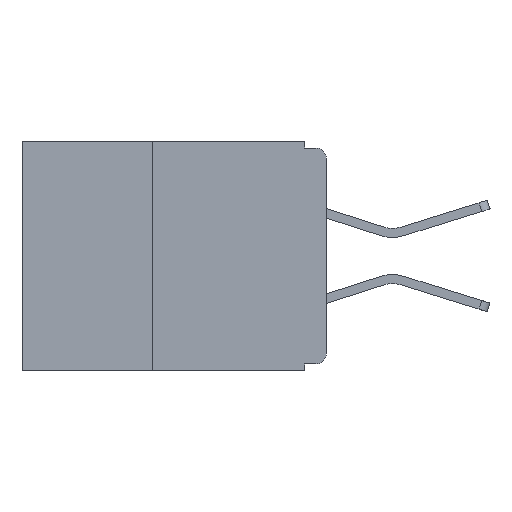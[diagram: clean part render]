
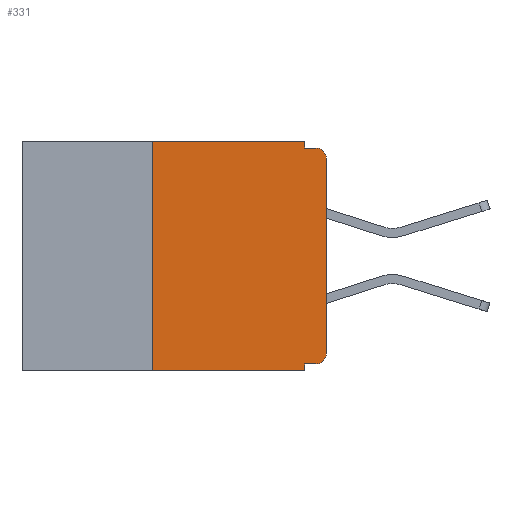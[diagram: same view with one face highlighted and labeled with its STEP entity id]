
A CAD part, left-side view. The second image highlights one B-rep face of the part: STEP entity #331.
In plain terms, the highlighted planar face has unit normal (-1, 0, 0).
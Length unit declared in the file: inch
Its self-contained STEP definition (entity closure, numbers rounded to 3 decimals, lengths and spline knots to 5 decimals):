
#97 = ORIENTED_EDGE ( 'NONE', *, *, #522, .F. ) ;
#331 = ADVANCED_FACE ( 'NONE', ( #19796 ), #12678, .F. ) ;
#342 = ORIENTED_EDGE ( 'NONE', *, *, #9798, .T. ) ;
#350 = VECTOR ( 'NONE', #2283, 39.37008 ) ;
#358 = EDGE_LOOP ( 'NONE', ( #603, #11187, #97, #20735, #12195, #6514, #342, #10022, #10660, #18268 ) ) ;
#522 = EDGE_CURVE ( 'NONE', #19656, #4964, #21245, .T. ) ;
#603 = ORIENTED_EDGE ( 'NONE', *, *, #3829, .T. ) ;
#1118 = CARTESIAN_POINT ( 'NONE',  ( 0., 0., -0.32 ) ) ;
#2044 = VECTOR ( 'NONE', #4149, 39.37008 ) ;
#2244 = CARTESIAN_POINT ( 'NONE',  ( 0., 0.25, -0.33 ) ) ;
#2283 = DIRECTION ( 'NONE',  ( 0., 0., -1. ) ) ;
#2284 = VERTEX_POINT ( 'NONE', #16833 ) ;
#2367 = VECTOR ( 'NONE', #20820, 39.37008 ) ;
#2995 = DIRECTION ( 'NONE',  ( 0., 1., 0. ) ) ;
#3829 = EDGE_CURVE ( 'NONE', #8977, #16353, #7368, .T. ) ;
#3917 = CARTESIAN_POINT ( 'NONE',  ( 0., 0.015, -0.305 ) ) ;
#4149 = DIRECTION ( 'NONE',  ( 0., 0., 1. ) ) ;
#4964 = VERTEX_POINT ( 'NONE', #22934 ) ;
#5152 = VECTOR ( 'NONE', #16269, 39.37008 ) ;
#5301 = VERTEX_POINT ( 'NONE', #5804 ) ;
#5392 = CARTESIAN_POINT ( 'NONE',  ( 0., 0.031, 0. ) ) ;
#5720 = LINE ( 'NONE', #10609, #20074 ) ;
#5778 = DIRECTION ( 'NONE',  ( 0., 0., -1. ) ) ;
#5804 = CARTESIAN_POINT ( 'NONE',  ( 0., 0.031, -0.33 ) ) ;
#5842 = CARTESIAN_POINT ( 'NONE',  ( 0., 0., -0.025 ) ) ;
#6514 = ORIENTED_EDGE ( 'NONE', *, *, #10430, .F. ) ;
#6812 = EDGE_CURVE ( 'NONE', #2284, #11528, #15078, .T. ) ;
#7368 = LINE ( 'NONE', #10387, #16692 ) ;
#7522 = VERTEX_POINT ( 'NONE', #18755 ) ;
#7772 = CARTESIAN_POINT ( 'NONE',  ( 0., 0.437, -0.33 ) ) ;
#8536 = CARTESIAN_POINT ( 'NONE',  ( 0., 0.015, -0.025 ) ) ;
#8763 = DIRECTION ( 'NONE',  ( 0., 0., -1. ) ) ;
#8977 = VERTEX_POINT ( 'NONE', #22898 ) ;
#9481 = EDGE_CURVE ( 'NONE', #16353, #4964, #14965, .T. ) ;
#9701 = VERTEX_POINT ( 'NONE', #12780 ) ;
#9798 = EDGE_CURVE ( 'NONE', #17469, #5301, #12342, .T. ) ;
#9914 = DIRECTION ( 'NONE',  ( 0., 0., -1. ) ) ;
#9920 = DIRECTION ( 'NONE',  ( 1., 0., 0. ) ) ;
#10022 = ORIENTED_EDGE ( 'NONE', *, *, #15241, .F. ) ;
#10387 = CARTESIAN_POINT ( 'NONE',  ( 0., 0., 0. ) ) ;
#10406 = DIRECTION ( 'NONE',  ( 0., 0., -1. ) ) ;
#10430 = EDGE_CURVE ( 'NONE', #17469, #2284, #16940, .T. ) ;
#10609 = CARTESIAN_POINT ( 'NONE',  ( 0., 0.031, 0. ) ) ;
#10660 = ORIENTED_EDGE ( 'NONE', *, *, #12763, .F. ) ;
#11187 = ORIENTED_EDGE ( 'NONE', *, *, #9481, .T. ) ;
#11346 = VECTOR ( 'NONE', #18023, 39.37008 ) ;
#11528 = VERTEX_POINT ( 'NONE', #5392 ) ;
#12195 = ORIENTED_EDGE ( 'NONE', *, *, #6812, .F. ) ;
#12342 = LINE ( 'NONE', #7772, #2367 ) ;
#12678 = PLANE ( 'NONE',  #18622 ) ;
#12763 = EDGE_CURVE ( 'NONE', #7522, #9701, #21228, .T. ) ;
#12780 = CARTESIAN_POINT ( 'NONE',  ( 0., 0.031, -0.32 ) ) ;
#12805 = EDGE_CURVE ( 'NONE', #11528, #19656, #5720, .T. ) ;
#14474 = CARTESIAN_POINT ( 'NONE',  ( 0., 0.437, 0. ) ) ;
#14965 = CIRCLE ( 'NONE', #21642, 0.015 ) ;
#15078 = LINE ( 'NONE', #14474, #5152 ) ;
#15241 = EDGE_CURVE ( 'NONE', #9701, #5301, #20256, .T. ) ;
#16269 = DIRECTION ( 'NONE',  ( 0., -1., 0. ) ) ;
#16331 = CARTESIAN_POINT ( 'NONE',  ( 0., 0.437, 0. ) ) ;
#16353 = VERTEX_POINT ( 'NONE', #5842 ) ;
#16692 = VECTOR ( 'NONE', #21546, 39.37008 ) ;
#16795 = CIRCLE ( 'NONE', #17364, 0.015 ) ;
#16833 = CARTESIAN_POINT ( 'NONE',  ( 0., 0.25, 0. ) ) ;
#16940 = LINE ( 'NONE', #2244, #2044 ) ;
#16956 = DIRECTION ( 'NONE',  ( -1., 0., 0. ) ) ;
#17364 = AXIS2_PLACEMENT_3D ( 'NONE', #3917, #16956, #5778 ) ;
#17415 = VECTOR ( 'NONE', #2995, 39.37008 ) ;
#17469 = VERTEX_POINT ( 'NONE', #20261 ) ;
#18023 = DIRECTION ( 'NONE',  ( 0., -1., 0. ) ) ;
#18156 = CARTESIAN_POINT ( 'NONE',  ( 0., 0., -0.01 ) ) ;
#18268 = ORIENTED_EDGE ( 'NONE', *, *, #18664, .T. ) ;
#18622 = AXIS2_PLACEMENT_3D ( 'NONE', #16331, #9920, #9914 ) ;
#18664 = EDGE_CURVE ( 'NONE', #7522, #8977, #16795, .T. ) ;
#18755 = CARTESIAN_POINT ( 'NONE',  ( 0., 0.015, -0.32 ) ) ;
#19656 = VERTEX_POINT ( 'NONE', #20143 ) ;
#19796 = FACE_OUTER_BOUND ( 'NONE', #358, .T. ) ;
#20074 = VECTOR ( 'NONE', #8763, 39.37008 ) ;
#20143 = CARTESIAN_POINT ( 'NONE',  ( 0., 0.031, -0.01 ) ) ;
#20256 = LINE ( 'NONE', #20906, #350 ) ;
#20261 = CARTESIAN_POINT ( 'NONE',  ( 0., 0.25, -0.33 ) ) ;
#20735 = ORIENTED_EDGE ( 'NONE', *, *, #12805, .F. ) ;
#20820 = DIRECTION ( 'NONE',  ( 0., -1., 0. ) ) ;
#20906 = CARTESIAN_POINT ( 'NONE',  ( 0., 0.031, -0.33 ) ) ;
#21228 = LINE ( 'NONE', #1118, #17415 ) ;
#21245 = LINE ( 'NONE', #18156, #11346 ) ;
#21546 = DIRECTION ( 'NONE',  ( 0., 0., 1. ) ) ;
#21565 = DIRECTION ( 'NONE',  ( -1., 0., 0. ) ) ;
#21642 = AXIS2_PLACEMENT_3D ( 'NONE', #8536, #21565, #10406 ) ;
#22898 = CARTESIAN_POINT ( 'NONE',  ( 0., 0., -0.305 ) ) ;
#22934 = CARTESIAN_POINT ( 'NONE',  ( 0., 0.015, -0.01 ) ) ;
